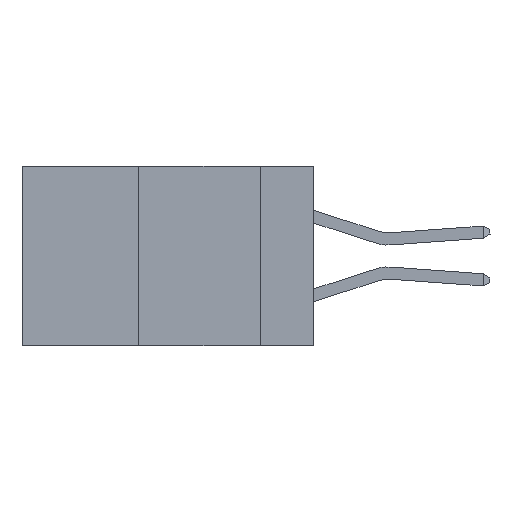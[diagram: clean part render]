
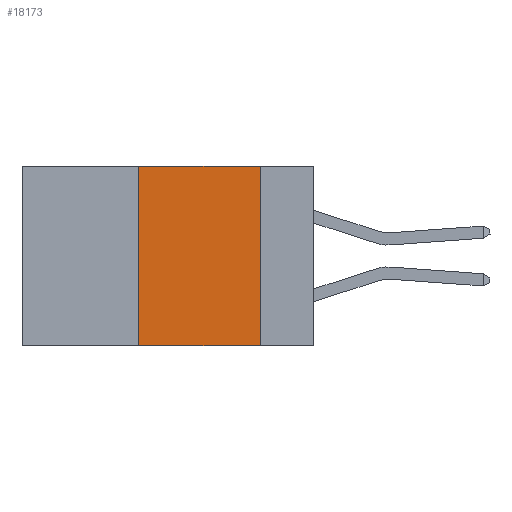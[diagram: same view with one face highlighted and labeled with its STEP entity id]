
A CAD part, left-side view. The second image highlights one B-rep face of the part: STEP entity #18173.
In plain terms, the highlighted planar face has unit normal (-1, 0, 0).
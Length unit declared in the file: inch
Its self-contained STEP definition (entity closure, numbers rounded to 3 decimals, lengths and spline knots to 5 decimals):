
#1446 = CARTESIAN_POINT ( 'NONE',  ( 0., 0.36, 0. ) ) ;
#1901 = DIRECTION ( 'NONE',  ( 0., -1., 0. ) ) ;
#2249 = VECTOR ( 'NONE', #1901, 39.37008 ) ;
#3137 = EDGE_LOOP ( 'NONE', ( #6323, #6047, #5251, #19456 ) ) ;
#3325 = VECTOR ( 'NONE', #5309, 39.37008 ) ;
#3540 = CARTESIAN_POINT ( 'NONE',  ( 0., 0.11, -0.37 ) ) ;
#3583 = CARTESIAN_POINT ( 'NONE',  ( 0., 0.36, -0.37 ) ) ;
#5083 = PLANE ( 'NONE',  #9370 ) ;
#5251 = ORIENTED_EDGE ( 'NONE', *, *, #5677, .F. ) ;
#5309 = DIRECTION ( 'NONE',  ( 0., 0., 1. ) ) ;
#5544 = LINE ( 'NONE', #6965, #18224 ) ;
#5669 = VERTEX_POINT ( 'NONE', #3583 ) ;
#5677 = EDGE_CURVE ( 'NONE', #5669, #16939, #11581, .T. ) ;
#6047 = ORIENTED_EDGE ( 'NONE', *, *, #12907, .F. ) ;
#6323 = ORIENTED_EDGE ( 'NONE', *, *, #12563, .F. ) ;
#6798 = FACE_OUTER_BOUND ( 'NONE', #3137, .T. ) ;
#6965 = CARTESIAN_POINT ( 'NONE',  ( 0., 0.11, 0. ) ) ;
#7996 = VECTOR ( 'NONE', #12951, 39.37008 ) ;
#8472 = DIRECTION ( 'NONE',  ( 0., 0., -1. ) ) ;
#9370 = AXIS2_PLACEMENT_3D ( 'NONE', #14411, #14212, #12986 ) ;
#10546 = VERTEX_POINT ( 'NONE', #12166 ) ;
#11581 = LINE ( 'NONE', #14632, #3325 ) ;
#12166 = CARTESIAN_POINT ( 'NONE',  ( 0., 0.11, 0. ) ) ;
#12563 = EDGE_CURVE ( 'NONE', #10546, #14075, #5544, .T. ) ;
#12731 = CARTESIAN_POINT ( 'NONE',  ( 0., 0.6, 0. ) ) ;
#12907 = EDGE_CURVE ( 'NONE', #16939, #10546, #15765, .T. ) ;
#12951 = DIRECTION ( 'NONE',  ( 0., -1., 0. ) ) ;
#12986 = DIRECTION ( 'NONE',  ( 0., 0., -1. ) ) ;
#14075 = VERTEX_POINT ( 'NONE', #3540 ) ;
#14109 = EDGE_CURVE ( 'NONE', #5669, #14075, #17494, .T. ) ;
#14212 = DIRECTION ( 'NONE',  ( 1., 0., 0. ) ) ;
#14411 = CARTESIAN_POINT ( 'NONE',  ( 0., 0.6, 0. ) ) ;
#14575 = CARTESIAN_POINT ( 'NONE',  ( 0., 0.6, -0.37 ) ) ;
#14632 = CARTESIAN_POINT ( 'NONE',  ( 0., 0.36, 0. ) ) ;
#15765 = LINE ( 'NONE', #12731, #2249 ) ;
#16939 = VERTEX_POINT ( 'NONE', #1446 ) ;
#17494 = LINE ( 'NONE', #14575, #7996 ) ;
#18173 = ADVANCED_FACE ( 'NONE', ( #6798 ), #5083, .F. ) ;
#18224 = VECTOR ( 'NONE', #8472, 39.37008 ) ;
#19456 = ORIENTED_EDGE ( 'NONE', *, *, #14109, .T. ) ;
